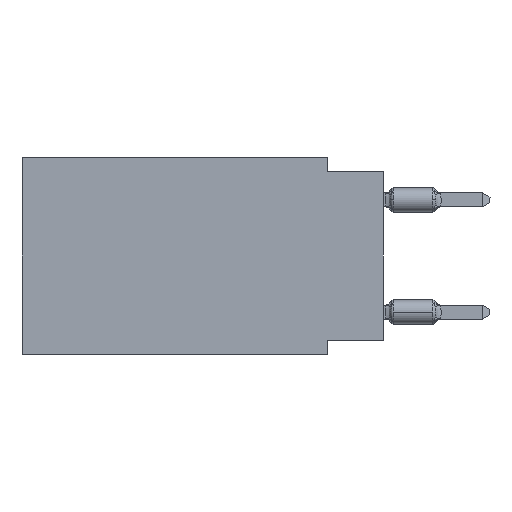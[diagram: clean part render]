
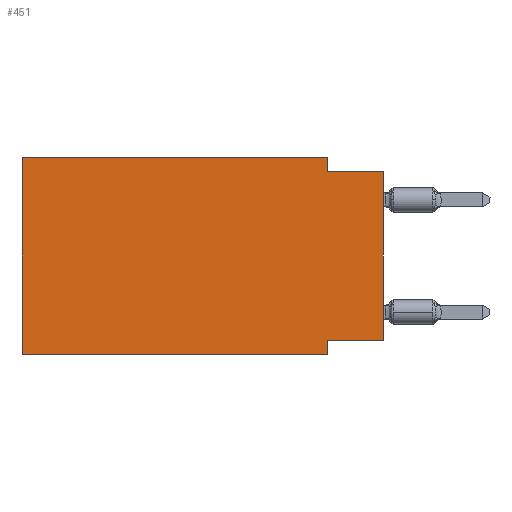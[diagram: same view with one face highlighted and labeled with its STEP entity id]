
A CAD part, left-side view. The second image highlights one B-rep face of the part: STEP entity #451.
In plain terms, the highlighted planar face has unit normal (-1, 0, 0).
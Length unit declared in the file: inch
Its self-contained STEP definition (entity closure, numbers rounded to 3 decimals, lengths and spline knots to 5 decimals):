
#121 = DIRECTION ( 'NONE',  ( 0., 0., 1. ) ) ;
#142 = LINE ( 'NONE', #8074, #1652 ) ;
#195 = CARTESIAN_POINT ( 'NONE',  ( 0., 0., -0.325 ) ) ;
#300 = ORIENTED_EDGE ( 'NONE', *, *, #11418, .T. ) ;
#451 = ADVANCED_FACE ( 'NONE', ( #9077 ), #11215, .F. ) ;
#698 = ORIENTED_EDGE ( 'NONE', *, *, #12604, .F. ) ;
#778 = DIRECTION ( 'NONE',  ( 0., 0., -1. ) ) ;
#946 = DIRECTION ( 'NONE',  ( 0., -1., 0. ) ) ;
#1188 = CARTESIAN_POINT ( 'NONE',  ( 0., 0.645, 0. ) ) ;
#1253 = ORIENTED_EDGE ( 'NONE', *, *, #7992, .F. ) ;
#1434 = CARTESIAN_POINT ( 'NONE',  ( 0., 0., -0.325 ) ) ;
#1652 = VECTOR ( 'NONE', #5798, 39.37008 ) ;
#1711 = CARTESIAN_POINT ( 'NONE',  ( 0., 0., -0.025 ) ) ;
#1907 = ORIENTED_EDGE ( 'NONE', *, *, #6984, .T. ) ;
#2292 = VECTOR ( 'NONE', #946, 39.37008 ) ;
#2329 = VERTEX_POINT ( 'NONE', #13011 ) ;
#2522 = VECTOR ( 'NONE', #7290, 39.37008 ) ;
#2563 = ORIENTED_EDGE ( 'NONE', *, *, #2780, .F. ) ;
#2600 = VERTEX_POINT ( 'NONE', #13834 ) ;
#2780 = EDGE_CURVE ( 'NONE', #11314, #5327, #10629, .T. ) ;
#2821 = CARTESIAN_POINT ( 'NONE',  ( 0., 0., 0. ) ) ;
#2952 = VERTEX_POINT ( 'NONE', #1711 ) ;
#3198 = CARTESIAN_POINT ( 'NONE',  ( 0., 0.1, -0.35 ) ) ;
#3331 = VERTEX_POINT ( 'NONE', #5568 ) ;
#4112 = CARTESIAN_POINT ( 'NONE',  ( 0., 0.1, 0. ) ) ;
#4361 = CARTESIAN_POINT ( 'NONE',  ( 0., 0., -0.025 ) ) ;
#4555 = LINE ( 'NONE', #1188, #7486 ) ;
#5261 = ORIENTED_EDGE ( 'NONE', *, *, #7136, .F. ) ;
#5327 = VERTEX_POINT ( 'NONE', #6556 ) ;
#5568 = CARTESIAN_POINT ( 'NONE',  ( 0., 0.645, 0. ) ) ;
#5572 = DIRECTION ( 'NONE',  ( 0., 0., -1. ) ) ;
#5798 = DIRECTION ( 'NONE',  ( 0., -1., 0. ) ) ;
#6254 = DIRECTION ( 'NONE',  ( 0., 0., -1. ) ) ;
#6417 = AXIS2_PLACEMENT_3D ( 'NONE', #13731, #14716, #778 ) ;
#6488 = DIRECTION ( 'NONE',  ( 0., 0., 1. ) ) ;
#6556 = CARTESIAN_POINT ( 'NONE',  ( 0., 0.1, -0.325 ) ) ;
#6798 = DIRECTION ( 'NONE',  ( 0., -1., 0. ) ) ;
#6864 = LINE ( 'NONE', #3198, #10596 ) ;
#6984 = EDGE_CURVE ( 'NONE', #2600, #7507, #142, .T. ) ;
#7030 = VERTEX_POINT ( 'NONE', #9354 ) ;
#7136 = EDGE_CURVE ( 'NONE', #2329, #7030, #7545, .T. ) ;
#7290 = DIRECTION ( 'NONE',  ( 0., 1., 0. ) ) ;
#7486 = VECTOR ( 'NONE', #121, 39.37008 ) ;
#7507 = VERTEX_POINT ( 'NONE', #7649 ) ;
#7545 = LINE ( 'NONE', #4112, #11746 ) ;
#7649 = CARTESIAN_POINT ( 'NONE',  ( 0., 0.1, -0.35 ) ) ;
#7693 = LINE ( 'NONE', #2821, #11815 ) ;
#7793 = ORIENTED_EDGE ( 'NONE', *, *, #9268, .F. ) ;
#7992 = EDGE_CURVE ( 'NONE', #7030, #2952, #14986, .T. ) ;
#8074 = CARTESIAN_POINT ( 'NONE',  ( 0., 0.645, -0.35 ) ) ;
#8759 = EDGE_LOOP ( 'NONE', ( #300, #1253, #5261, #7793, #698, #1907, #10724, #2563 ) ) ;
#9077 = FACE_OUTER_BOUND ( 'NONE', #8759, .T. ) ;
#9268 = EDGE_CURVE ( 'NONE', #3331, #2329, #14801, .T. ) ;
#9354 = CARTESIAN_POINT ( 'NONE',  ( 0., 0.1, -0.025 ) ) ;
#10596 = VECTOR ( 'NONE', #5572, 39.37008 ) ;
#10629 = LINE ( 'NONE', #195, #2522 ) ;
#10724 = ORIENTED_EDGE ( 'NONE', *, *, #11196, .F. ) ;
#11196 = EDGE_CURVE ( 'NONE', #5327, #7507, #6864, .T. ) ;
#11215 = PLANE ( 'NONE',  #6417 ) ;
#11314 = VERTEX_POINT ( 'NONE', #1434 ) ;
#11381 = CARTESIAN_POINT ( 'NONE',  ( 0., 0.645, 0. ) ) ;
#11418 = EDGE_CURVE ( 'NONE', #11314, #2952, #7693, .T. ) ;
#11746 = VECTOR ( 'NONE', #6254, 39.37008 ) ;
#11815 = VECTOR ( 'NONE', #6488, 39.37008 ) ;
#12604 = EDGE_CURVE ( 'NONE', #2600, #3331, #4555, .T. ) ;
#13011 = CARTESIAN_POINT ( 'NONE',  ( 0., 0.1, 0. ) ) ;
#13731 = CARTESIAN_POINT ( 'NONE',  ( 0., 0.645, 0. ) ) ;
#13734 = VECTOR ( 'NONE', #6798, 39.37008 ) ;
#13834 = CARTESIAN_POINT ( 'NONE',  ( 0., 0.645, -0.35 ) ) ;
#14716 = DIRECTION ( 'NONE',  ( 1., 0., 0. ) ) ;
#14801 = LINE ( 'NONE', #11381, #2292 ) ;
#14986 = LINE ( 'NONE', #4361, #13734 ) ;
